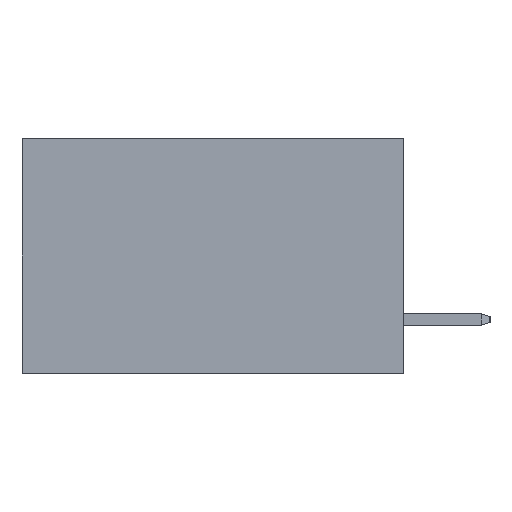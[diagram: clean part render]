
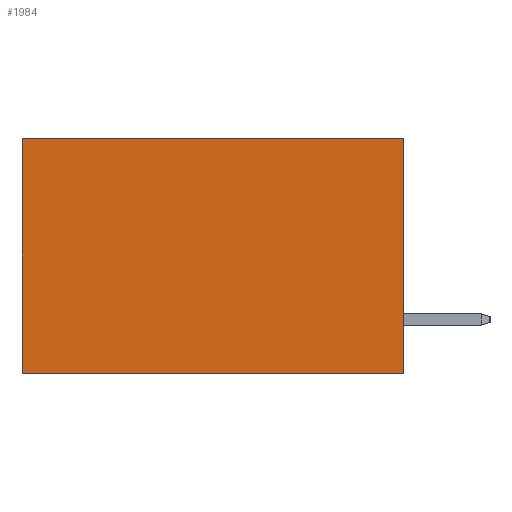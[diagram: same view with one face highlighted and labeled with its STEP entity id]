
A CAD part, left-side view. The second image highlights one B-rep face of the part: STEP entity #1984.
In plain terms, the highlighted planar face has unit normal (-1, 0, 0).
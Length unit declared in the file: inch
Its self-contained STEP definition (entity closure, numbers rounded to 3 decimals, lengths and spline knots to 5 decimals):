
#162 = CARTESIAN_POINT ( 'NONE',  ( 0.2875, 0.6, 0. ) ) ;
#222 = DIRECTION ( 'NONE',  ( 0., 0., -1. ) ) ;
#553 = CARTESIAN_POINT ( 'NONE',  ( 0.2875, 0., -0.37 ) ) ;
#630 = ORIENTED_EDGE ( 'NONE', *, *, #18282, .T. ) ;
#694 = PLANE ( 'NONE',  #14320 ) ;
#1250 = ORIENTED_EDGE ( 'NONE', *, *, #11280, .F. ) ;
#1984 = ADVANCED_FACE ( 'NONE', ( #8454 ), #694, .F. ) ;
#3266 = EDGE_LOOP ( 'NONE', ( #6050, #8785, #1250, #630 ) ) ;
#4511 = VERTEX_POINT ( 'NONE', #162 ) ;
#4838 = LINE ( 'NONE', #553, #16432 ) ;
#5573 = CARTESIAN_POINT ( 'NONE',  ( 0.2875, 0., 0. ) ) ;
#5660 = LINE ( 'NONE', #5573, #14092 ) ;
#5999 = CARTESIAN_POINT ( 'NONE',  ( 0.2875, 0.6, 0. ) ) ;
#6050 = ORIENTED_EDGE ( 'NONE', *, *, #19436, .T. ) ;
#8121 = DIRECTION ( 'NONE',  ( 0., 1., 0. ) ) ;
#8454 = FACE_OUTER_BOUND ( 'NONE', #3266, .T. ) ;
#8785 = ORIENTED_EDGE ( 'NONE', *, *, #13240, .F. ) ;
#9189 = VERTEX_POINT ( 'NONE', #18511 ) ;
#11280 = EDGE_CURVE ( 'NONE', #14894, #17979, #5660, .T. ) ;
#11534 = DIRECTION ( 'NONE',  ( 1., 0., 0. ) ) ;
#13220 = DIRECTION ( 'NONE',  ( 0., 0., -1. ) ) ;
#13240 = EDGE_CURVE ( 'NONE', #17979, #9189, #4838, .T. ) ;
#13858 = LINE ( 'NONE', #5999, #18163 ) ;
#14092 = VECTOR ( 'NONE', #13220, 39.37008 ) ;
#14320 = AXIS2_PLACEMENT_3D ( 'NONE', #15801, #11534, #16092 ) ;
#14531 = DIRECTION ( 'NONE',  ( 0., 1., 0. ) ) ;
#14666 = CARTESIAN_POINT ( 'NONE',  ( 0.2875, 0., 0. ) ) ;
#14894 = VERTEX_POINT ( 'NONE', #14666 ) ;
#15801 = CARTESIAN_POINT ( 'NONE',  ( 0.2875, 0., 0. ) ) ;
#16092 = DIRECTION ( 'NONE',  ( 0., 0., -1. ) ) ;
#16208 = CARTESIAN_POINT ( 'NONE',  ( 0.2875, 0., 0. ) ) ;
#16318 = LINE ( 'NONE', #16208, #17532 ) ;
#16432 = VECTOR ( 'NONE', #8121, 39.37008 ) ;
#17532 = VECTOR ( 'NONE', #14531, 39.37008 ) ;
#17979 = VERTEX_POINT ( 'NONE', #19343 ) ;
#18163 = VECTOR ( 'NONE', #222, 39.37008 ) ;
#18282 = EDGE_CURVE ( 'NONE', #14894, #4511, #16318, .T. ) ;
#18511 = CARTESIAN_POINT ( 'NONE',  ( 0.2875, 0.6, -0.37 ) ) ;
#19343 = CARTESIAN_POINT ( 'NONE',  ( 0.2875, 0., -0.37 ) ) ;
#19436 = EDGE_CURVE ( 'NONE', #4511, #9189, #13858, .T. ) ;
